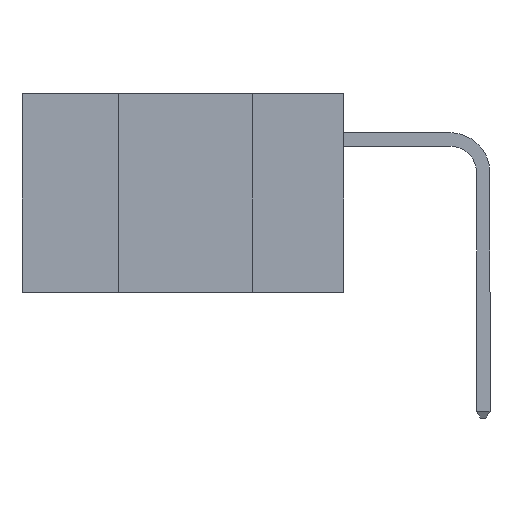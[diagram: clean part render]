
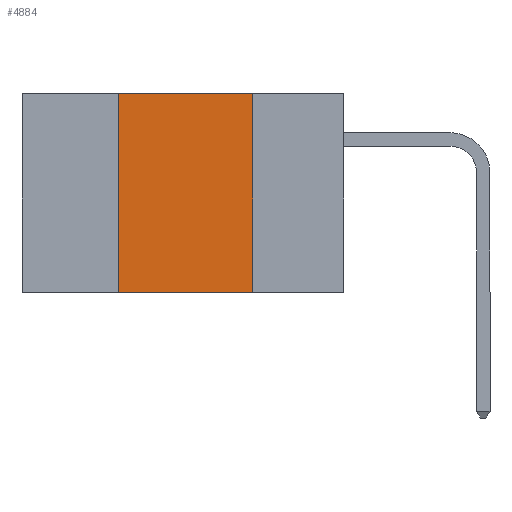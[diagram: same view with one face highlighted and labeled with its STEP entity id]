
A CAD part, left-side view. The second image highlights one B-rep face of the part: STEP entity #4884.
In plain terms, the highlighted planar face has unit normal (-1, 0, 0).
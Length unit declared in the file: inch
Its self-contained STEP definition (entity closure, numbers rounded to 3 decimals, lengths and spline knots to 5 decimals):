
#77 = VECTOR ( 'NONE', #768, 39.37008 ) ;
#331 = LINE ( 'NONE', #631, #77 ) ;
#491 = AXIS2_PLACEMENT_3D ( 'NONE', #4732, #8421, #8428 ) ;
#589 = CARTESIAN_POINT ( 'NONE',  ( 0., 0.17, -0.37 ) ) ;
#613 = EDGE_CURVE ( 'NONE', #2021, #4425, #4149, .T. ) ;
#631 = CARTESIAN_POINT ( 'NONE',  ( 0., 0.17, 0. ) ) ;
#768 = DIRECTION ( 'NONE',  ( 0., 0., -1. ) ) ;
#1092 = CARTESIAN_POINT ( 'NONE',  ( 0., 0.6, -0.37 ) ) ;
#1189 = CARTESIAN_POINT ( 'NONE',  ( 0., 0.42, 0. ) ) ;
#1562 = EDGE_LOOP ( 'NONE', ( #2787, #6934, #3613, #6259 ) ) ;
#1757 = CARTESIAN_POINT ( 'NONE',  ( 0., 0.17, 0. ) ) ;
#2021 = VERTEX_POINT ( 'NONE', #1189 ) ;
#2040 = VECTOR ( 'NONE', #4451, 39.37008 ) ;
#2139 = DIRECTION ( 'NONE',  ( 0., -1., 0. ) ) ;
#2547 = VERTEX_POINT ( 'NONE', #5927 ) ;
#2787 = ORIENTED_EDGE ( 'NONE', *, *, #6729, .F. ) ;
#2989 = VECTOR ( 'NONE', #2139, 39.37008 ) ;
#3613 = ORIENTED_EDGE ( 'NONE', *, *, #8894, .F. ) ;
#3685 = VECTOR ( 'NONE', #7406, 39.37008 ) ;
#4149 = LINE ( 'NONE', #7426, #2040 ) ;
#4425 = VERTEX_POINT ( 'NONE', #1757 ) ;
#4451 = DIRECTION ( 'NONE',  ( 0., -1., 0. ) ) ;
#4732 = CARTESIAN_POINT ( 'NONE',  ( 0., 0.6, 0. ) ) ;
#4884 = ADVANCED_FACE ( 'NONE', ( #8347 ), #5081, .F. ) ;
#5081 = PLANE ( 'NONE',  #491 ) ;
#5927 = CARTESIAN_POINT ( 'NONE',  ( 0., 0.42, -0.37 ) ) ;
#6259 = ORIENTED_EDGE ( 'NONE', *, *, #6296, .T. ) ;
#6296 = EDGE_CURVE ( 'NONE', #2547, #7518, #7092, .T. ) ;
#6729 = EDGE_CURVE ( 'NONE', #4425, #7518, #331, .T. ) ;
#6748 = CARTESIAN_POINT ( 'NONE',  ( 0., 0.42, 0. ) ) ;
#6934 = ORIENTED_EDGE ( 'NONE', *, *, #613, .F. ) ;
#7092 = LINE ( 'NONE', #1092, #2989 ) ;
#7406 = DIRECTION ( 'NONE',  ( 0., 0., 1. ) ) ;
#7426 = CARTESIAN_POINT ( 'NONE',  ( 0., 0.6, 0. ) ) ;
#7518 = VERTEX_POINT ( 'NONE', #589 ) ;
#8347 = FACE_OUTER_BOUND ( 'NONE', #1562, .T. ) ;
#8421 = DIRECTION ( 'NONE',  ( 1., 0., 0. ) ) ;
#8428 = DIRECTION ( 'NONE',  ( 0., 0., -1. ) ) ;
#8894 = EDGE_CURVE ( 'NONE', #2547, #2021, #9657, .T. ) ;
#9657 = LINE ( 'NONE', #6748, #3685 ) ;
